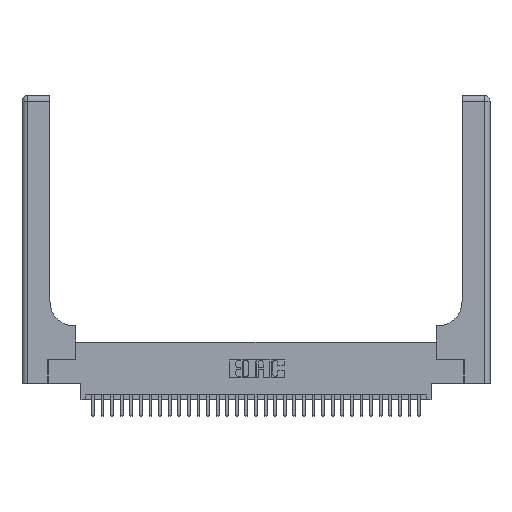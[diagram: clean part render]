
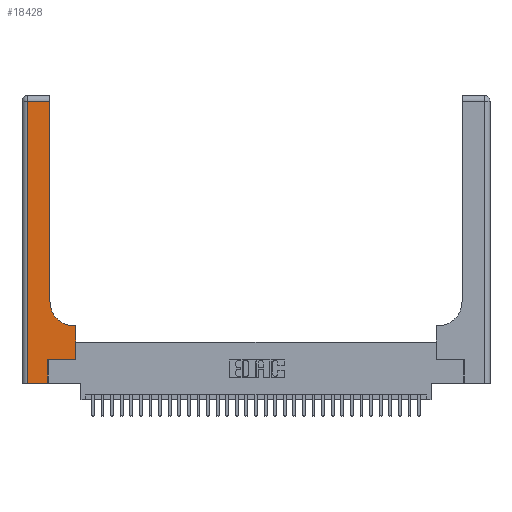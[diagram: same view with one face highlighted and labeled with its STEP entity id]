
A CAD part, top view. The second image highlights one B-rep face of the part: STEP entity #18428.
In plain terms, the highlighted planar face has unit normal (0, 0, 1).
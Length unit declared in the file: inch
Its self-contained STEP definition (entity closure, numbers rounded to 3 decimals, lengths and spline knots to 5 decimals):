
#593 = VECTOR ( 'NONE', #13888, 39.37008 ) ;
#764 = LINE ( 'NONE', #949, #30268 ) ;
#949 = CARTESIAN_POINT ( 'NONE',  ( 0., 0., 0.37 ) ) ;
#950 = DIRECTION ( 'NONE',  ( 0., 0., -1. ) ) ;
#1350 = DIRECTION ( 'NONE',  ( 0., 0., -1. ) ) ;
#2142 = ORIENTED_EDGE ( 'NONE', *, *, #7875, .T. ) ;
#2694 = CARTESIAN_POINT ( 'NONE',  ( 0.2915, 2.94, 0.37 ) ) ;
#2997 = CARTESIAN_POINT ( 'NONE',  ( 0.269, 0., 0.37 ) ) ;
#3157 = VECTOR ( 'NONE', #31572, 39.37008 ) ;
#3657 = VERTEX_POINT ( 'NONE', #18437 ) ;
#3666 = VERTEX_POINT ( 'NONE', #2997 ) ;
#4158 = ORIENTED_EDGE ( 'NONE', *, *, #11425, .T. ) ;
#4462 = ORIENTED_EDGE ( 'NONE', *, *, #18194, .T. ) ;
#5904 = EDGE_CURVE ( 'NONE', #7798, #8344, #8923, .T. ) ;
#6916 = VERTEX_POINT ( 'NONE', #14104 ) ;
#7798 = VERTEX_POINT ( 'NONE', #8792 ) ;
#7875 = EDGE_CURVE ( 'NONE', #30880, #7798, #28395, .T. ) ;
#8344 = VERTEX_POINT ( 'NONE', #2694 ) ;
#8488 = LINE ( 'NONE', #15914, #3157 ) ;
#8792 = CARTESIAN_POINT ( 'NONE',  ( 0.2915, 0.85, 0.37 ) ) ;
#8923 = LINE ( 'NONE', #25687, #10544 ) ;
#9459 = CARTESIAN_POINT ( 'NONE',  ( 0.06, 2.94, 0.37 ) ) ;
#9960 = FACE_OUTER_BOUND ( 'NONE', #30105, .T. ) ;
#10011 = CARTESIAN_POINT ( 'NONE',  ( 0.269, 0.25, 0.37 ) ) ;
#10544 = VECTOR ( 'NONE', #17589, 39.37008 ) ;
#11425 = EDGE_CURVE ( 'NONE', #3657, #3666, #764, .T. ) ;
#11667 = CARTESIAN_POINT ( 'NONE',  ( 0.5415, 0.6, 0.37 ) ) ;
#12013 = LINE ( 'NONE', #29551, #593 ) ;
#13680 = ORIENTED_EDGE ( 'NONE', *, *, #17891, .T. ) ;
#13888 = DIRECTION ( 'NONE',  ( 0., 1., 0. ) ) ;
#14099 = DIRECTION ( 'NONE',  ( 0., -1., 0. ) ) ;
#14104 = CARTESIAN_POINT ( 'NONE',  ( 0.5585, 0.6, 0.37 ) ) ;
#14105 = CARTESIAN_POINT ( 'NONE',  ( 0.2915, 0.6, 0.37 ) ) ;
#15291 = ORIENTED_EDGE ( 'NONE', *, *, #5904, .T. ) ;
#15914 = CARTESIAN_POINT ( 'NONE',  ( 0., 2.94, 0.37 ) ) ;
#16444 = EDGE_CURVE ( 'NONE', #8344, #30013, #8488, .T. ) ;
#16897 = CARTESIAN_POINT ( 'NONE',  ( 0.5585, 0.25, 0.37 ) ) ;
#17589 = DIRECTION ( 'NONE',  ( 0., 1., 0. ) ) ;
#17891 = EDGE_CURVE ( 'NONE', #3666, #31636, #12013, .T. ) ;
#18194 = EDGE_CURVE ( 'NONE', #24335, #6916, #23463, .T. ) ;
#18428 = ADVANCED_FACE ( 'NONE', ( #9960 ), #26992, .F. ) ;
#18437 = CARTESIAN_POINT ( 'NONE',  ( 0.06, 0., 0.37 ) ) ;
#19332 = ORIENTED_EDGE ( 'NONE', *, *, #16444, .T. ) ;
#19406 = CARTESIAN_POINT ( 'NONE',  ( 0.5415, 0.85, 0.37 ) ) ;
#19451 = CARTESIAN_POINT ( 'NONE',  ( 0., 3., 0.37 ) ) ;
#19474 = DIRECTION ( 'NONE',  ( -1., 0., 0. ) ) ;
#20200 = DIRECTION ( 'NONE',  ( 1., 0., 0. ) ) ;
#20904 = EDGE_CURVE ( 'NONE', #31636, #24335, #31103, .T. ) ;
#21388 = ORIENTED_EDGE ( 'NONE', *, *, #25480, .T. ) ;
#22040 = DIRECTION ( 'NONE',  ( 1., 0., 0. ) ) ;
#23243 = DIRECTION ( 'NONE',  ( 0., 1., 0. ) ) ;
#23401 = LINE ( 'NONE', #32477, #23746 ) ;
#23463 = LINE ( 'NONE', #30795, #33711 ) ;
#23746 = VECTOR ( 'NONE', #14099, 39.37008 ) ;
#24335 = VERTEX_POINT ( 'NONE', #16897 ) ;
#25085 = AXIS2_PLACEMENT_3D ( 'NONE', #19451, #950, #29757 ) ;
#25480 = EDGE_CURVE ( 'NONE', #30013, #3657, #23401, .T. ) ;
#25687 = CARTESIAN_POINT ( 'NONE',  ( 0.2915, 3., 0.37 ) ) ;
#25967 = VECTOR ( 'NONE', #19474, 39.37008 ) ;
#26386 = EDGE_CURVE ( 'NONE', #6916, #30880, #30930, .T. ) ;
#26992 = PLANE ( 'NONE',  #25085 ) ;
#27118 = AXIS2_PLACEMENT_3D ( 'NONE', #19406, #1350, #22040 ) ;
#28395 = CIRCLE ( 'NONE', #27118, 0.25 ) ;
#28640 = ORIENTED_EDGE ( 'NONE', *, *, #26386, .T. ) ;
#29551 = CARTESIAN_POINT ( 'NONE',  ( 0.269, 0., 0.37 ) ) ;
#29756 = DIRECTION ( 'NONE',  ( 1., 0., 0. ) ) ;
#29757 = DIRECTION ( 'NONE',  ( -1., 0., 0. ) ) ;
#30013 = VERTEX_POINT ( 'NONE', #9459 ) ;
#30105 = EDGE_LOOP ( 'NONE', ( #15291, #19332, #21388, #4158, #13680, #30612, #4462, #28640, #2142 ) ) ;
#30268 = VECTOR ( 'NONE', #29756, 39.37008 ) ;
#30612 = ORIENTED_EDGE ( 'NONE', *, *, #20904, .T. ) ;
#30795 = CARTESIAN_POINT ( 'NONE',  ( 0.5585, 0.25, 0.37 ) ) ;
#30880 = VERTEX_POINT ( 'NONE', #11667 ) ;
#30930 = LINE ( 'NONE', #14105, #25967 ) ;
#31103 = LINE ( 'NONE', #10011, #33564 ) ;
#31123 = CARTESIAN_POINT ( 'NONE',  ( 0.269, 0.25, 0.37 ) ) ;
#31572 = DIRECTION ( 'NONE',  ( -1., 0., 0. ) ) ;
#31636 = VERTEX_POINT ( 'NONE', #31123 ) ;
#32477 = CARTESIAN_POINT ( 'NONE',  ( 0.06, 3., 0.37 ) ) ;
#33564 = VECTOR ( 'NONE', #20200, 39.37008 ) ;
#33711 = VECTOR ( 'NONE', #23243, 39.37008 ) ;
